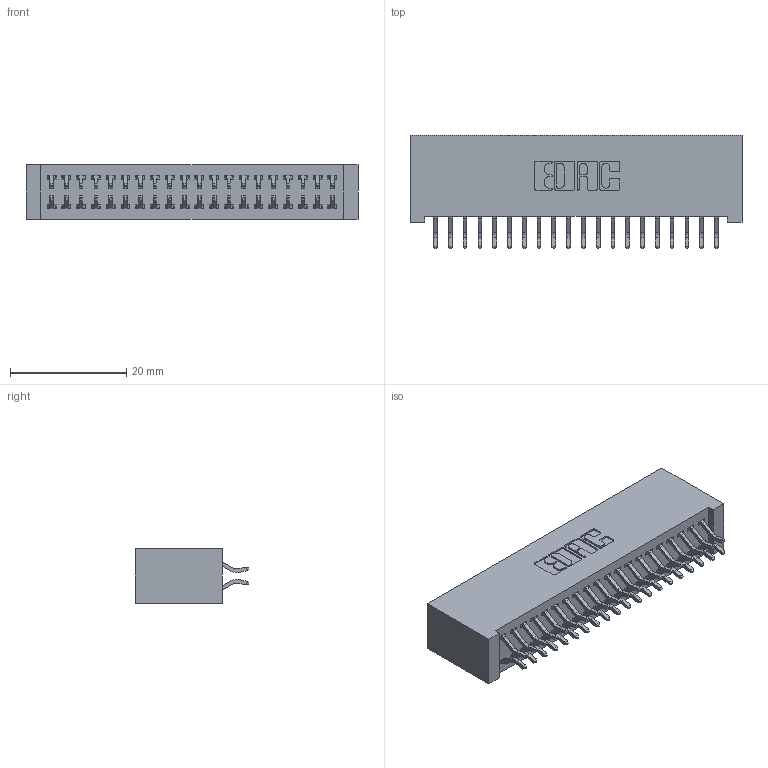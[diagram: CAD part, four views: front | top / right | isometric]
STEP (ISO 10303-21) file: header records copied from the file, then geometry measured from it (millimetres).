
FILE_DESCRIPTION (( 'STEP AP203' ), '1' );
FILE_NAME ('342-040-556-201.STEP', '2019-10-02T16:59:55', ( '' ), ( '' ), 'SwSTEP 2.0', 'SolidWorks 2016', '' );
FILE_SCHEMA (( 'CONFIG_CONTROL_DESIGN' ));
Length unit declared in the file: inch
Products named in the file (3): 342 Part_Lugless; 345-292-001_556 Tail; 342-040-556-201
Assembly tree (41 placements, depth 2):
  342-040-556-201
    342 Part_Lugless
    345-292-001_556 Tail  x40
Bounding box: 57.05 x 19.58 x 9.4 mm (x, y, z)
Volume: 5460.2 mm3; surface area: 8753.1 mm2
Topology: 41 solids, 41 shells, 2422 faces, 7195 edges, 4742 vertices
Faces by surface type: plane 1662, cylinder 760
Entity records: 15523 total; most frequent: CARTESIAN_POINT 2610, ORIENTED_EDGE 2534, DIRECTION 2251, EDGE_CURVE 1267, LINE 1139, VECTOR 1139, VERTEX_POINT 842, AXIS2_PLACEMENT_3D 556
